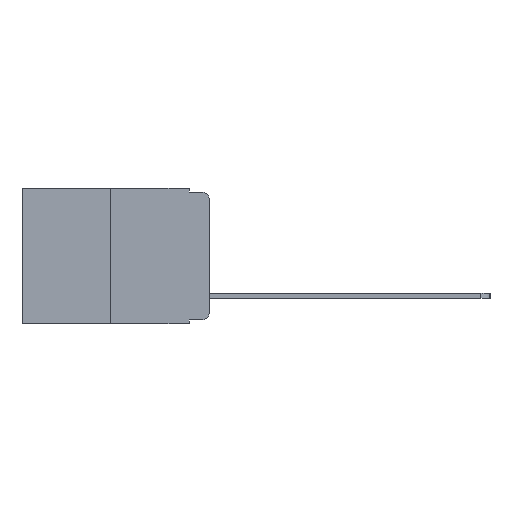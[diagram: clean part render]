
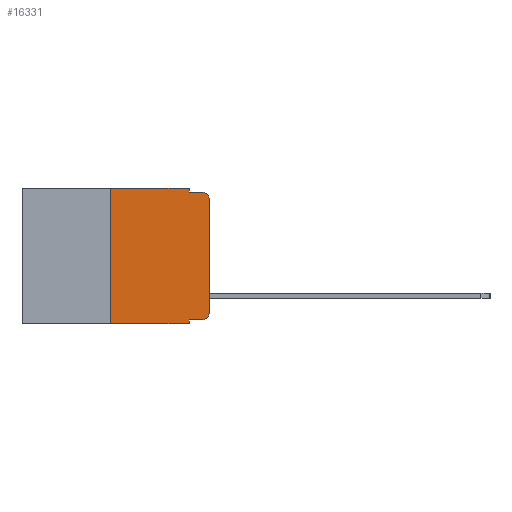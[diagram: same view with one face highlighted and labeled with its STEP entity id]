
A CAD part, left-side view. The second image highlights one B-rep face of the part: STEP entity #16331.
In plain terms, the highlighted planar face has unit normal (-1, 0, 0).
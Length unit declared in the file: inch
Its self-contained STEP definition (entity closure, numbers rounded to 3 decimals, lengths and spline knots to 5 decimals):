
#267 = CARTESIAN_POINT ( 'NONE',  ( 0., 0.473, 0. ) ) ;
#364 = VERTEX_POINT ( 'NONE', #16686 ) ;
#391 = DIRECTION ( 'NONE',  ( 0., 0., -1. ) ) ;
#677 = EDGE_CURVE ( 'NONE', #2459, #2022, #1349, .T. ) ;
#777 = LINE ( 'NONE', #6550, #12912 ) ;
#982 = EDGE_CURVE ( 'NONE', #4621, #10478, #12718, .T. ) ;
#1163 = VERTEX_POINT ( 'NONE', #7459 ) ;
#1212 = DIRECTION ( 'NONE',  ( -1., 0., 0. ) ) ;
#1349 = CIRCLE ( 'NONE', #19753, 0.02 ) ;
#1400 = ORIENTED_EDGE ( 'NONE', *, *, #19747, .F. ) ;
#1524 = DIRECTION ( 'NONE',  ( 0., 0., -1. ) ) ;
#1648 = DIRECTION ( 'NONE',  ( 0., 0., 1. ) ) ;
#1768 = EDGE_CURVE ( 'NONE', #364, #2459, #10471, .T. ) ;
#1936 = DIRECTION ( 'NONE',  ( 0., -1., 0. ) ) ;
#2022 = VERTEX_POINT ( 'NONE', #6188 ) ;
#2051 = VECTOR ( 'NONE', #1648, 39.37008 ) ;
#2307 = CARTESIAN_POINT ( 'NONE',  ( 0., 0.051, 0. ) ) ;
#2459 = VERTEX_POINT ( 'NONE', #2563 ) ;
#2563 = CARTESIAN_POINT ( 'NONE',  ( 0., 0., -0.03 ) ) ;
#2660 = LINE ( 'NONE', #8339, #10563 ) ;
#2881 = VERTEX_POINT ( 'NONE', #17026 ) ;
#3433 = VECTOR ( 'NONE', #19271, 39.37008 ) ;
#4092 = VERTEX_POINT ( 'NONE', #2307 ) ;
#4349 = ORIENTED_EDGE ( 'NONE', *, *, #8543, .T. ) ;
#4621 = VERTEX_POINT ( 'NONE', #11901 ) ;
#5085 = ORIENTED_EDGE ( 'NONE', *, *, #15773, .F. ) ;
#5324 = CARTESIAN_POINT ( 'NONE',  ( 0., 0.051, -0.01 ) ) ;
#6115 = DIRECTION ( 'NONE',  ( 0., 0., 1. ) ) ;
#6188 = CARTESIAN_POINT ( 'NONE',  ( 0., 0.02, -0.01 ) ) ;
#6550 = CARTESIAN_POINT ( 'NONE',  ( 0., 0.051, 0. ) ) ;
#6662 = VECTOR ( 'NONE', #17644, 39.37008 ) ;
#6844 = EDGE_LOOP ( 'NONE', ( #11146, #9256, #1400, #5085, #13275, #15459, #18217, #11404, #13456, #4349 ) ) ;
#6929 = CIRCLE ( 'NONE', #16188, 0.02 ) ;
#6973 = VECTOR ( 'NONE', #1936, 39.37008 ) ;
#7302 = DIRECTION ( 'NONE',  ( -1., 0., 0. ) ) ;
#7424 = VERTEX_POINT ( 'NONE', #13912 ) ;
#7459 = CARTESIAN_POINT ( 'NONE',  ( 0., 0.02, -0.333 ) ) ;
#7636 = EDGE_CURVE ( 'NONE', #7424, #4092, #7940, .T. ) ;
#7655 = LINE ( 'NONE', #5324, #6662 ) ;
#7831 = CARTESIAN_POINT ( 'NONE',  ( 0., 0.473, 0. ) ) ;
#7940 = LINE ( 'NONE', #267, #6973 ) ;
#8127 = DIRECTION ( 'NONE',  ( 0., 0., -1. ) ) ;
#8339 = CARTESIAN_POINT ( 'NONE',  ( 0., 0.051, 0. ) ) ;
#8543 = EDGE_CURVE ( 'NONE', #1163, #364, #6929, .T. ) ;
#9014 = VECTOR ( 'NONE', #9321, 39.37008 ) ;
#9198 = CARTESIAN_POINT ( 'NONE',  ( 0., 0.25, 0. ) ) ;
#9256 = ORIENTED_EDGE ( 'NONE', *, *, #677, .T. ) ;
#9321 = DIRECTION ( 'NONE',  ( 0., -1., 0. ) ) ;
#9604 = EDGE_CURVE ( 'NONE', #2881, #1163, #15831, .T. ) ;
#10303 = DIRECTION ( 'NONE',  ( 0., 0., -1. ) ) ;
#10471 = LINE ( 'NONE', #17528, #2051 ) ;
#10478 = VERTEX_POINT ( 'NONE', #12280 ) ;
#10563 = VECTOR ( 'NONE', #391, 39.37008 ) ;
#11010 = DIRECTION ( 'NONE',  ( 1., 0., 0. ) ) ;
#11146 = ORIENTED_EDGE ( 'NONE', *, *, #1768, .T. ) ;
#11404 = ORIENTED_EDGE ( 'NONE', *, *, #13779, .F. ) ;
#11901 = CARTESIAN_POINT ( 'NONE',  ( 0., 0.25, -0.343 ) ) ;
#12280 = CARTESIAN_POINT ( 'NONE',  ( 0., 0.051, -0.343 ) ) ;
#12718 = LINE ( 'NONE', #19627, #9014 ) ;
#12912 = VECTOR ( 'NONE', #8127, 39.37008 ) ;
#13207 = LINE ( 'NONE', #9198, #19705 ) ;
#13275 = ORIENTED_EDGE ( 'NONE', *, *, #7636, .F. ) ;
#13456 = ORIENTED_EDGE ( 'NONE', *, *, #9604, .T. ) ;
#13779 = EDGE_CURVE ( 'NONE', #2881, #10478, #2660, .T. ) ;
#13912 = CARTESIAN_POINT ( 'NONE',  ( 0., 0.25, 0. ) ) ;
#13984 = PLANE ( 'NONE',  #17787 ) ;
#14777 = EDGE_CURVE ( 'NONE', #4621, #7424, #13207, .T. ) ;
#15143 = CARTESIAN_POINT ( 'NONE',  ( 0., 0.051, -0.01 ) ) ;
#15459 = ORIENTED_EDGE ( 'NONE', *, *, #14777, .F. ) ;
#15773 = EDGE_CURVE ( 'NONE', #4092, #18803, #777, .T. ) ;
#15831 = LINE ( 'NONE', #17806, #3433 ) ;
#16188 = AXIS2_PLACEMENT_3D ( 'NONE', #16547, #7302, #18033 ) ;
#16331 = ADVANCED_FACE ( 'NONE', ( #18748 ), #13984, .F. ) ;
#16547 = CARTESIAN_POINT ( 'NONE',  ( 0., 0.02, -0.313 ) ) ;
#16686 = CARTESIAN_POINT ( 'NONE',  ( 0., 0., -0.313 ) ) ;
#17026 = CARTESIAN_POINT ( 'NONE',  ( 0., 0.051, -0.333 ) ) ;
#17528 = CARTESIAN_POINT ( 'NONE',  ( 0., 0., 0. ) ) ;
#17644 = DIRECTION ( 'NONE',  ( 0., -1., 0. ) ) ;
#17787 = AXIS2_PLACEMENT_3D ( 'NONE', #7831, #11010, #1524 ) ;
#17806 = CARTESIAN_POINT ( 'NONE',  ( 0., 0.051, -0.333 ) ) ;
#18033 = DIRECTION ( 'NONE',  ( 0., 0., -1. ) ) ;
#18217 = ORIENTED_EDGE ( 'NONE', *, *, #982, .T. ) ;
#18748 = FACE_OUTER_BOUND ( 'NONE', #6844, .T. ) ;
#18803 = VERTEX_POINT ( 'NONE', #15143 ) ;
#19271 = DIRECTION ( 'NONE',  ( 0., -1., 0. ) ) ;
#19303 = CARTESIAN_POINT ( 'NONE',  ( 0., 0.02, -0.03 ) ) ;
#19627 = CARTESIAN_POINT ( 'NONE',  ( 0., 0.473, -0.343 ) ) ;
#19705 = VECTOR ( 'NONE', #6115, 39.37008 ) ;
#19747 = EDGE_CURVE ( 'NONE', #18803, #2022, #7655, .T. ) ;
#19753 = AXIS2_PLACEMENT_3D ( 'NONE', #19303, #1212, #10303 ) ;
